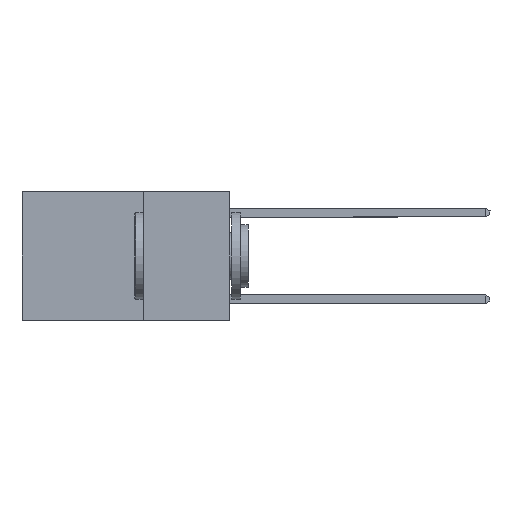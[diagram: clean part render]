
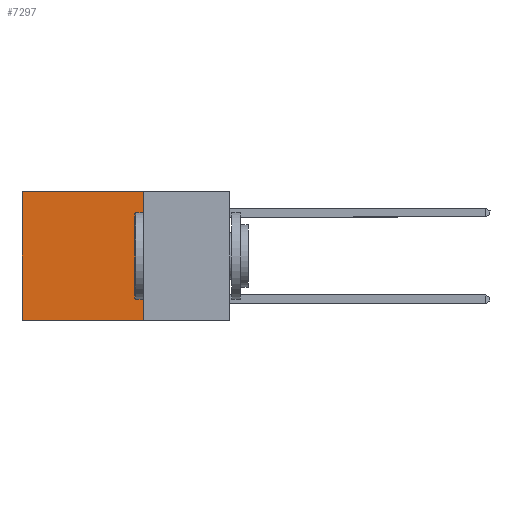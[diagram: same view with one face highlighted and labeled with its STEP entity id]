
A CAD part, left-side view. The second image highlights one B-rep face of the part: STEP entity #7297.
In plain terms, the highlighted planar face has unit normal (-1, 0, 0).
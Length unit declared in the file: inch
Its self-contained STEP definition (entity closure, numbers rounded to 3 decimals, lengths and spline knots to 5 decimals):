
#43 = EDGE_CURVE ( 'NONE', #8933, #2153, #5147, .T. ) ;
#599 = DIRECTION ( 'NONE',  ( 0., 1., 0. ) ) ;
#694 = LINE ( 'NONE', #11635, #10072 ) ;
#703 = VECTOR ( 'NONE', #3323, 39.37008 ) ;
#1046 = EDGE_CURVE ( 'NONE', #4365, #8933, #3177, .T. ) ;
#1199 = LINE ( 'NONE', #3362, #10009 ) ;
#1434 = EDGE_CURVE ( 'NONE', #5796, #2153, #694, .T. ) ;
#1686 = PLANE ( 'NONE',  #4025 ) ;
#2153 = VERTEX_POINT ( 'NONE', #11373 ) ;
#2624 = DIRECTION ( 'NONE',  ( 1., 0., 0. ) ) ;
#3177 = LINE ( 'NONE', #3777, #703 ) ;
#3323 = DIRECTION ( 'NONE',  ( 0., 0., -1. ) ) ;
#3348 = CARTESIAN_POINT ( 'NONE',  ( 0.2625, 0.25, -0.37 ) ) ;
#3362 = CARTESIAN_POINT ( 'NONE',  ( 0.2625, 0.25, 0. ) ) ;
#3777 = CARTESIAN_POINT ( 'NONE',  ( 0.2625, 0.25, 0. ) ) ;
#4025 = AXIS2_PLACEMENT_3D ( 'NONE', #9794, #2624, #8952 ) ;
#4263 = CARTESIAN_POINT ( 'NONE',  ( 0.2625, 0.6, 0. ) ) ;
#4365 = VERTEX_POINT ( 'NONE', #10876 ) ;
#5147 = LINE ( 'NONE', #3348, #6968 ) ;
#5796 = VERTEX_POINT ( 'NONE', #4263 ) ;
#6087 = EDGE_LOOP ( 'NONE', ( #11365, #11445, #11553, #11565 ) ) ;
#6968 = VECTOR ( 'NONE', #11269, 39.37008 ) ;
#7181 = FACE_OUTER_BOUND ( 'NONE', #6087, .T. ) ;
#7297 = ADVANCED_FACE ( 'NONE', ( #7181 ), #1686, .F. ) ;
#7503 = CARTESIAN_POINT ( 'NONE',  ( 0.2625, 0.25, -0.37 ) ) ;
#8051 = EDGE_CURVE ( 'NONE', #4365, #5796, #1199, .T. ) ;
#8933 = VERTEX_POINT ( 'NONE', #7503 ) ;
#8952 = DIRECTION ( 'NONE',  ( 0., 0., -1. ) ) ;
#9123 = DIRECTION ( 'NONE',  ( 0., 0., -1. ) ) ;
#9794 = CARTESIAN_POINT ( 'NONE',  ( 0.2625, 0.25, 0. ) ) ;
#10009 = VECTOR ( 'NONE', #599, 39.37008 ) ;
#10072 = VECTOR ( 'NONE', #9123, 39.37008 ) ;
#10876 = CARTESIAN_POINT ( 'NONE',  ( 0.2625, 0.25, 0. ) ) ;
#11269 = DIRECTION ( 'NONE',  ( 0., 1., 0. ) ) ;
#11365 = ORIENTED_EDGE ( 'NONE', *, *, #1434, .T. ) ;
#11373 = CARTESIAN_POINT ( 'NONE',  ( 0.2625, 0.6, -0.37 ) ) ;
#11445 = ORIENTED_EDGE ( 'NONE', *, *, #43, .F. ) ;
#11553 = ORIENTED_EDGE ( 'NONE', *, *, #1046, .F. ) ;
#11565 = ORIENTED_EDGE ( 'NONE', *, *, #8051, .T. ) ;
#11635 = CARTESIAN_POINT ( 'NONE',  ( 0.2625, 0.6, 0. ) ) ;
